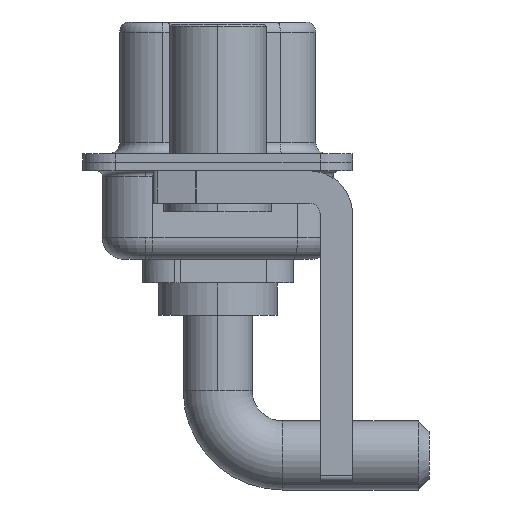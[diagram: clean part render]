
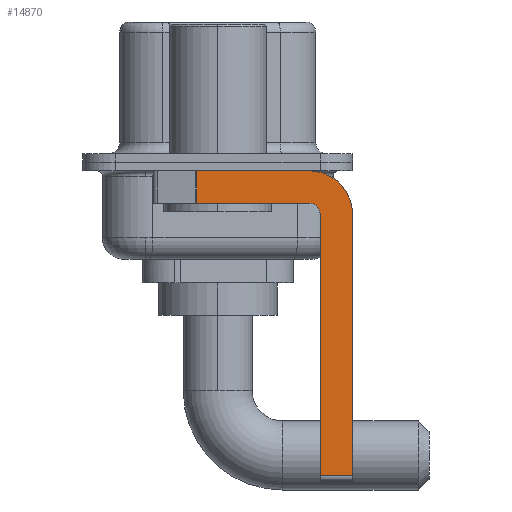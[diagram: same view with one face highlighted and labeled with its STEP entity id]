
A CAD part, left-side view. The second image highlights one B-rep face of the part: STEP entity #14870.
In plain terms, the highlighted planar face has unit normal (-1, 0, 0).
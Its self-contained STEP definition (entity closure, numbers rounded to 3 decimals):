
#55 = DIRECTION ( 'NONE',  ( 0., 1., 0. ) ) ;
#328 = VECTOR ( 'NONE', #6642, 1000. ) ;
#353 = ORIENTED_EDGE ( 'NONE', *, *, #12511, .F. ) ;
#649 = DIRECTION ( 'NONE',  ( 1., 0., 0. ) ) ;
#1709 = CARTESIAN_POINT ( 'NONE',  ( -2.9, -4.75, -2.4 ) ) ;
#2172 = VERTEX_POINT ( 'NONE', #11761 ) ;
#2297 = EDGE_CURVE ( 'NONE', #6057, #12874, #14349, .T. ) ;
#2337 = LINE ( 'NONE', #10194, #13170 ) ;
#2505 = ORIENTED_EDGE ( 'NONE', *, *, #10504, .F. ) ;
#2571 = CARTESIAN_POINT ( 'NONE',  ( -2.9, 0.978, -1.9 ) ) ;
#2858 = VECTOR ( 'NONE', #14546, 1000. ) ;
#2978 = CARTESIAN_POINT ( 'NONE',  ( -2.9, -4.75, -14.8 ) ) ;
#3005 = CARTESIAN_POINT ( 'NONE',  ( -2.9, -6.25, -14.55 ) ) ;
#3034 = PLANE ( 'NONE',  #8814 ) ;
#3125 = CARTESIAN_POINT ( 'NONE',  ( -2.9, -4.25, -2.4 ) ) ;
#3160 = ORIENTED_EDGE ( 'NONE', *, *, #5286, .F. ) ;
#3202 = VERTEX_POINT ( 'NONE', #3005 ) ;
#3941 = DIRECTION ( 'NONE',  ( 0., 0., 1. ) ) ;
#4285 = VECTOR ( 'NONE', #55, 1000. ) ;
#4400 = CARTESIAN_POINT ( 'NONE',  ( -2.9, 0.978, -0.4 ) ) ;
#4489 = FACE_OUTER_BOUND ( 'NONE', #12311, .T. ) ;
#5286 = EDGE_CURVE ( 'NONE', #14904, #16605, #2337, .T. ) ;
#5924 = DIRECTION ( 'NONE',  ( 1., 0., 0. ) ) ;
#6057 = VERTEX_POINT ( 'NONE', #12135 ) ;
#6083 = VERTEX_POINT ( 'NONE', #1709 ) ;
#6642 = DIRECTION ( 'NONE',  ( 0., 0., 1. ) ) ;
#6931 = CARTESIAN_POINT ( 'NONE',  ( -2.9, -4.75, -14.55 ) ) ;
#6994 = CARTESIAN_POINT ( 'NONE',  ( -2.9, -4.25, -14.55 ) ) ;
#7340 = AXIS2_PLACEMENT_3D ( 'NONE', #13002, #15652, #3941 ) ;
#7472 = ORIENTED_EDGE ( 'NONE', *, *, #15749, .T. ) ;
#8440 = CIRCLE ( 'NONE', #7340, 0.5 ) ;
#8814 = AXIS2_PLACEMENT_3D ( 'NONE', #3125, #649, #13563 ) ;
#9022 = LINE ( 'NONE', #14253, #15018 ) ;
#9640 = LINE ( 'NONE', #6994, #2858 ) ;
#9981 = EDGE_CURVE ( 'NONE', #6083, #6057, #8440, .T. ) ;
#10194 = CARTESIAN_POINT ( 'NONE',  ( -2.9, 3., -0.4 ) ) ;
#10221 = EDGE_CURVE ( 'NONE', #16792, #6083, #13158, .T. ) ;
#10504 = EDGE_CURVE ( 'NONE', #2172, #3202, #9022, .T. ) ;
#11761 = CARTESIAN_POINT ( 'NONE',  ( -2.9, -6.25, -2.4 ) ) ;
#11765 = CIRCLE ( 'NONE', #15606, 2. ) ;
#12135 = CARTESIAN_POINT ( 'NONE',  ( -2.9, -4.25, -1.9 ) ) ;
#12311 = EDGE_LOOP ( 'NONE', ( #3160, #13513, #12546, #15617, #13040, #7472, #2505, #353 ) ) ;
#12511 = EDGE_CURVE ( 'NONE', #16605, #2172, #11765, .T. ) ;
#12546 = ORIENTED_EDGE ( 'NONE', *, *, #2297, .F. ) ;
#12874 = VERTEX_POINT ( 'NONE', #13926 ) ;
#12921 = LINE ( 'NONE', #2571, #16519 ) ;
#13002 = CARTESIAN_POINT ( 'NONE',  ( -2.9, -4.25, -2.4 ) ) ;
#13040 = ORIENTED_EDGE ( 'NONE', *, *, #10221, .F. ) ;
#13065 = CARTESIAN_POINT ( 'NONE',  ( -2.9, -4.25, -1.9 ) ) ;
#13158 = LINE ( 'NONE', #2978, #328 ) ;
#13170 = VECTOR ( 'NONE', #15347, 1000. ) ;
#13362 = CARTESIAN_POINT ( 'NONE',  ( -2.9, -4.25, -0.4 ) ) ;
#13513 = ORIENTED_EDGE ( 'NONE', *, *, #15620, .T. ) ;
#13563 = DIRECTION ( 'NONE',  ( 0., 0., -1. ) ) ;
#13809 = DIRECTION ( 'NONE',  ( 0., 0., -1. ) ) ;
#13926 = CARTESIAN_POINT ( 'NONE',  ( -2.9, 0.978, -1.9 ) ) ;
#14167 = DIRECTION ( 'NONE',  ( 0., 0., -1. ) ) ;
#14253 = CARTESIAN_POINT ( 'NONE',  ( -2.9, -6.25, -2.4 ) ) ;
#14349 = LINE ( 'NONE', #13065, #4285 ) ;
#14457 = DIRECTION ( 'NONE',  ( 0., 0., -1. ) ) ;
#14546 = DIRECTION ( 'NONE',  ( 0., -1., 0. ) ) ;
#14870 = ADVANCED_FACE ( 'NONE', ( #4489 ), #3034, .F. ) ;
#14904 = VERTEX_POINT ( 'NONE', #4400 ) ;
#14931 = CARTESIAN_POINT ( 'NONE',  ( -2.9, -4.25, -2.4 ) ) ;
#15018 = VECTOR ( 'NONE', #14167, 1000. ) ;
#15347 = DIRECTION ( 'NONE',  ( 0., -1., 0. ) ) ;
#15606 = AXIS2_PLACEMENT_3D ( 'NONE', #14931, #5924, #13809 ) ;
#15617 = ORIENTED_EDGE ( 'NONE', *, *, #9981, .F. ) ;
#15620 = EDGE_CURVE ( 'NONE', #14904, #12874, #12921, .T. ) ;
#15652 = DIRECTION ( 'NONE',  ( -1., 0., 0. ) ) ;
#15749 = EDGE_CURVE ( 'NONE', #16792, #3202, #9640, .T. ) ;
#16519 = VECTOR ( 'NONE', #14457, 1000. ) ;
#16605 = VERTEX_POINT ( 'NONE', #13362 ) ;
#16792 = VERTEX_POINT ( 'NONE', #6931 ) ;
